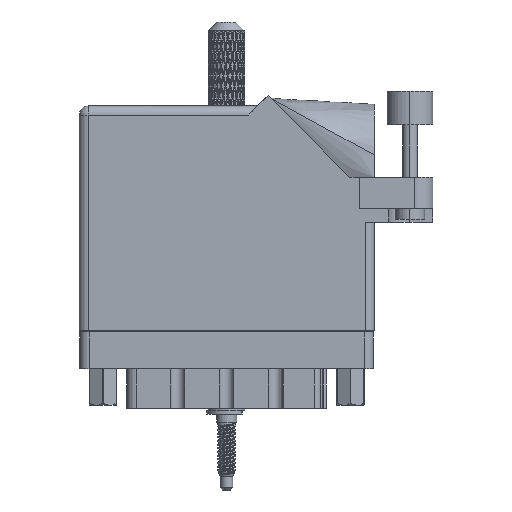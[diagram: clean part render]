
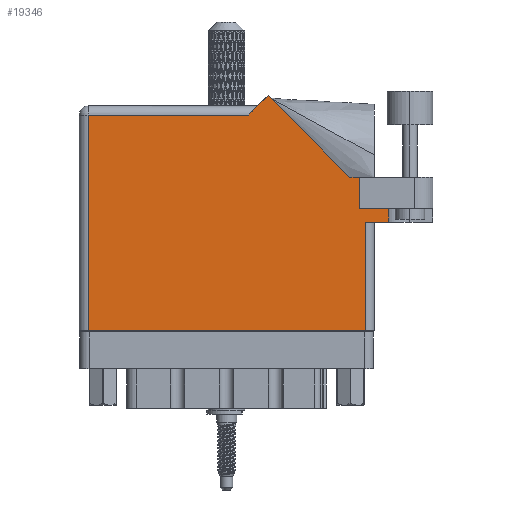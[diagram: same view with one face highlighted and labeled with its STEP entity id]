
A CAD part, front view. The second image highlights one B-rep face of the part: STEP entity #19346.
In plain terms, the highlighted face is planar.
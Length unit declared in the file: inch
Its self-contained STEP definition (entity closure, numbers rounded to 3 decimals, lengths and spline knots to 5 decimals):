
#223 = EDGE_CURVE ( 'NONE', #59177, #36935, #110051, .T. ) ;
#566 = DIRECTION ( 'NONE',  ( 1., 0., 0. ) ) ;
#1506 = VERTEX_POINT ( 'NONE', #104174 ) ;
#2004 = VERTEX_POINT ( 'NONE', #74632 ) ;
#3662 = VECTOR ( 'NONE', #90725, 39.37008 ) ;
#6825 = DIRECTION ( 'NONE',  ( -1., 0., 0. ) ) ;
#7575 = LINE ( 'NONE', #69759, #83022 ) ;
#7898 = ORIENTED_EDGE ( 'NONE', *, *, #65992, .T. ) ;
#8615 = EDGE_CURVE ( 'NONE', #36935, #2004, #52311, .T. ) ;
#13864 = ORIENTED_EDGE ( 'NONE', *, *, #20475, .T. ) ;
#14023 = EDGE_CURVE ( 'NONE', #83976, #29577, #26472, .T. ) ;
#15105 = CARTESIAN_POINT ( 'NONE',  ( 2.1115, 0.831, 0. ) ) ;
#17660 = CARTESIAN_POINT ( 'NONE',  ( 1.91, 1.044, 0. ) ) ;
#19268 = CARTESIAN_POINT ( 'NONE',  ( 2.41, 1.044, 0. ) ) ;
#19346 = ADVANCED_FACE ( 'NONE', ( #59373 ), #33389, .F. ) ;
#19846 = EDGE_CURVE ( 'NONE', #29577, #1506, #7575, .T. ) ;
#20475 = EDGE_CURVE ( 'NONE', #59004, #58469, #112423, .T. ) ;
#24239 = CARTESIAN_POINT ( 'NONE',  ( 1.948, 0.737, 0. ) ) ;
#25251 = ORIENTED_EDGE ( 'NONE', *, *, #69811, .T. ) ;
#26472 = LINE ( 'NONE', #100008, #97760 ) ;
#26784 = ORIENTED_EDGE ( 'NONE', *, *, #104028, .T. ) ;
#29577 = VERTEX_POINT ( 'NONE', #35694 ) ;
#29935 = LINE ( 'NONE', #36435, #73144 ) ;
#30135 = ORIENTED_EDGE ( 'NONE', *, *, #8615, .F. ) ;
#33243 = DIRECTION ( 'NONE',  ( 0., 1., 0. ) ) ;
#33336 = VECTOR ( 'NONE', #64144, 39.37008 ) ;
#33389 = PLANE ( 'NONE',  #55224 ) ;
#34854 = DIRECTION ( 'NONE',  ( 0., -1., 0. ) ) ;
#35694 = CARTESIAN_POINT ( 'NONE',  ( 1.155, 1.468, 0. ) ) ;
#36435 = CARTESIAN_POINT ( 'NONE',  ( 1.91, 0.831, 0. ) ) ;
#36723 = CARTESIAN_POINT ( 'NONE',  ( 1.84442, 1.044, 0. ) ) ;
#36935 = VERTEX_POINT ( 'NONE', #15105 ) ;
#40526 = LINE ( 'NONE', #24239, #113201 ) ;
#44664 = VECTOR ( 'NONE', #34854, 39.37008 ) ;
#45844 = CARTESIAN_POINT ( 'NONE',  ( 1.91, 0.831, 0. ) ) ;
#48104 = CARTESIAN_POINT ( 'NONE',  ( 0., 0., 0. ) ) ;
#50559 = DIRECTION ( 'NONE',  ( -0.707, -0.707, 0. ) ) ;
#52311 = LINE ( 'NONE', #104063, #73149 ) ;
#52420 = DIRECTION ( 'NONE',  ( 0., 0., -1. ) ) ;
#55224 = AXIS2_PLACEMENT_3D ( 'NONE', #60614, #52420, #115045 ) ;
#55357 = ORIENTED_EDGE ( 'NONE', *, *, #88662, .T. ) ;
#56139 = LINE ( 'NONE', #36723, #77050 ) ;
#58469 = VERTEX_POINT ( 'NONE', #83469 ) ;
#59004 = VERTEX_POINT ( 'NONE', #102477 ) ;
#59177 = VERTEX_POINT ( 'NONE', #64048 ) ;
#59373 = FACE_OUTER_BOUND ( 'NONE', #72892, .T. ) ;
#59813 = LINE ( 'NONE', #19268, #33336 ) ;
#60601 = VECTOR ( 'NONE', #74985, 39.37008 ) ;
#60614 = CARTESIAN_POINT ( 'NONE',  ( 0., 1.53, 0. ) ) ;
#62489 = VERTEX_POINT ( 'NONE', #17660 ) ;
#62803 = CARTESIAN_POINT ( 'NONE',  ( 0.062, 0., 0. ) ) ;
#64023 = EDGE_CURVE ( 'NONE', #92572, #83976, #56139, .T. ) ;
#64048 = CARTESIAN_POINT ( 'NONE',  ( 1.91, 0.831, 0. ) ) ;
#64144 = DIRECTION ( 'NONE',  ( -1., 0., 0. ) ) ;
#65992 = EDGE_CURVE ( 'NONE', #58469, #109288, #40526, .T. ) ;
#66924 = VECTOR ( 'NONE', #566, 39.37008 ) ;
#69746 = CARTESIAN_POINT ( 'NONE',  ( 1.84442, 1.044, 0. ) ) ;
#69759 = CARTESIAN_POINT ( 'NONE',  ( 0., 1.468, 0. ) ) ;
#69811 = EDGE_CURVE ( 'NONE', #109288, #2004, #100574, .T. ) ;
#70080 = ORIENTED_EDGE ( 'NONE', *, *, #14023, .T. ) ;
#71311 = EDGE_CURVE ( 'NONE', #1506, #59004, #73967, .T. ) ;
#72892 = EDGE_LOOP ( 'NONE', ( #13864, #7898, #25251, #30135, #87127, #55357, #26784, #111707, #70080, #95008, #91395 ) ) ;
#73144 = VECTOR ( 'NONE', #80058, 39.37008 ) ;
#73149 = VECTOR ( 'NONE', #112379, 39.37008 ) ;
#73967 = LINE ( 'NONE', #62803, #44664 ) ;
#74632 = CARTESIAN_POINT ( 'NONE',  ( 2.1115, 0.737, 0. ) ) ;
#74985 = DIRECTION ( 'NONE',  ( 1., 0., 0. ) ) ;
#77050 = VECTOR ( 'NONE', #82284, 39.37008 ) ;
#80058 = DIRECTION ( 'NONE',  ( 0., 1., 0. ) ) ;
#81455 = CARTESIAN_POINT ( 'NONE',  ( 2.01, 0.737, 0. ) ) ;
#82284 = DIRECTION ( 'NONE',  ( -0.707, 0.707, 0. ) ) ;
#83022 = VECTOR ( 'NONE', #6825, 39.37008 ) ;
#83469 = CARTESIAN_POINT ( 'NONE',  ( 1.948, 0., 0. ) ) ;
#83976 = VERTEX_POINT ( 'NONE', #98645 ) ;
#87127 = ORIENTED_EDGE ( 'NONE', *, *, #223, .F. ) ;
#88662 = EDGE_CURVE ( 'NONE', #59177, #62489, #29935, .T. ) ;
#90725 = DIRECTION ( 'NONE',  ( 1., 0., 0. ) ) ;
#91395 = ORIENTED_EDGE ( 'NONE', *, *, #71311, .T. ) ;
#92572 = VERTEX_POINT ( 'NONE', #69746 ) ;
#95008 = ORIENTED_EDGE ( 'NONE', *, *, #19846, .T. ) ;
#97760 = VECTOR ( 'NONE', #50559, 39.37008 ) ;
#98354 = CARTESIAN_POINT ( 'NONE',  ( 1.948, 0.737, 0. ) ) ;
#98645 = CARTESIAN_POINT ( 'NONE',  ( 1.28771, 1.60071, 0. ) ) ;
#100008 = CARTESIAN_POINT ( 'NONE',  ( 1.217, 1.53, 0. ) ) ;
#100574 = LINE ( 'NONE', #81455, #66924 ) ;
#102477 = CARTESIAN_POINT ( 'NONE',  ( 0.062, 0., 0. ) ) ;
#104028 = EDGE_CURVE ( 'NONE', #62489, #92572, #59813, .T. ) ;
#104063 = CARTESIAN_POINT ( 'NONE',  ( 2.1115, 1.16177, 0. ) ) ;
#104174 = CARTESIAN_POINT ( 'NONE',  ( 0.062, 1.468, 0. ) ) ;
#109288 = VERTEX_POINT ( 'NONE', #98354 ) ;
#110051 = LINE ( 'NONE', #45844, #3662 ) ;
#111707 = ORIENTED_EDGE ( 'NONE', *, *, #64023, .T. ) ;
#112379 = DIRECTION ( 'NONE',  ( 0., -1., 0. ) ) ;
#112423 = LINE ( 'NONE', #48104, #60601 ) ;
#113201 = VECTOR ( 'NONE', #33243, 39.37008 ) ;
#115045 = DIRECTION ( 'NONE',  ( -1., 0., 0. ) ) ;
